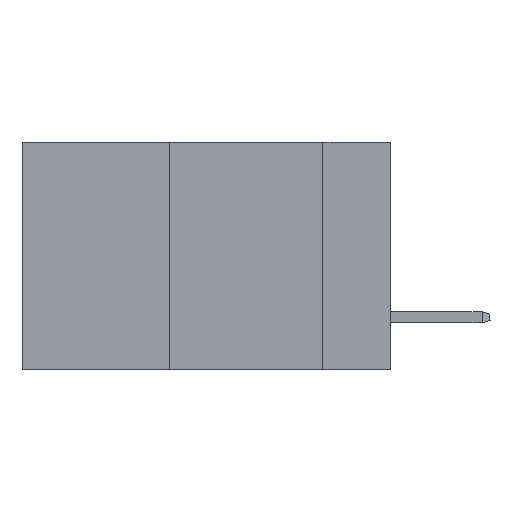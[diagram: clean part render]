
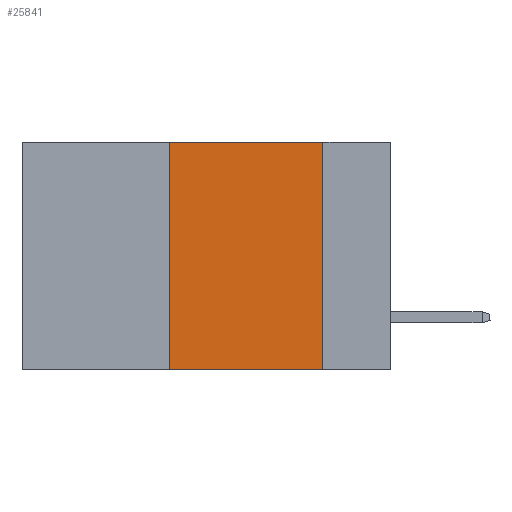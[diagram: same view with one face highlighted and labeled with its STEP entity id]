
A CAD part, left-side view. The second image highlights one B-rep face of the part: STEP entity #25841.
In plain terms, the highlighted planar face has unit normal (-1, 0, 0).
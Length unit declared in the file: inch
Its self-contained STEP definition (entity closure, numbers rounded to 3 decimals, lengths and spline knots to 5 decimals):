
#938 = VECTOR ( 'NONE', #4371, 39.37008 ) ;
#3241 = CARTESIAN_POINT ( 'NONE',  ( 0., 0.36, 0. ) ) ;
#4371 = DIRECTION ( 'NONE',  ( 0., 0., 1. ) ) ;
#6216 = VERTEX_POINT ( 'NONE', #20646 ) ;
#8365 = DIRECTION ( 'NONE',  ( 0., -1., 0. ) ) ;
#10169 = VECTOR ( 'NONE', #24412, 39.37008 ) ;
#11395 = EDGE_CURVE ( 'NONE', #15567, #6216, #29521, .T. ) ;
#13046 = DIRECTION ( 'NONE',  ( 1., 0., 0. ) ) ;
#13505 = VERTEX_POINT ( 'NONE', #3241 ) ;
#14642 = VECTOR ( 'NONE', #37794, 39.37008 ) ;
#14935 = VERTEX_POINT ( 'NONE', #39691 ) ;
#15514 = CARTESIAN_POINT ( 'NONE',  ( 0., 0.6, 0. ) ) ;
#15567 = VERTEX_POINT ( 'NONE', #29729 ) ;
#18575 = EDGE_CURVE ( 'NONE', #14935, #6216, #44314, .T. ) ;
#19691 = VECTOR ( 'NONE', #8365, 39.37008 ) ;
#20646 = CARTESIAN_POINT ( 'NONE',  ( 0., 0.11, -0.37 ) ) ;
#23724 = FACE_OUTER_BOUND ( 'NONE', #37494, .T. ) ;
#24412 = DIRECTION ( 'NONE',  ( 0., -1., 0. ) ) ;
#25841 = ADVANCED_FACE ( 'NONE', ( #23724 ), #41802, .F. ) ;
#29521 = LINE ( 'NONE', #46261, #10169 ) ;
#29678 = CARTESIAN_POINT ( 'NONE',  ( 0., 0.36, 0. ) ) ;
#29729 = CARTESIAN_POINT ( 'NONE',  ( 0., 0.36, -0.37 ) ) ;
#30243 = CARTESIAN_POINT ( 'NONE',  ( 0., 0.11, 0. ) ) ;
#31321 = ORIENTED_EDGE ( 'NONE', *, *, #11395, .T. ) ;
#33709 = ORIENTED_EDGE ( 'NONE', *, *, #39020, .F. ) ;
#34845 = EDGE_CURVE ( 'NONE', #13505, #14935, #40925, .T. ) ;
#37494 = EDGE_LOOP ( 'NONE', ( #37722, #41736, #33709, #31321 ) ) ;
#37722 = ORIENTED_EDGE ( 'NONE', *, *, #18575, .F. ) ;
#37794 = DIRECTION ( 'NONE',  ( 0., 0., -1. ) ) ;
#39020 = EDGE_CURVE ( 'NONE', #15567, #13505, #40318, .T. ) ;
#39691 = CARTESIAN_POINT ( 'NONE',  ( 0., 0.11, 0. ) ) ;
#40318 = LINE ( 'NONE', #29678, #938 ) ;
#40925 = LINE ( 'NONE', #15514, #19691 ) ;
#41736 = ORIENTED_EDGE ( 'NONE', *, *, #34845, .F. ) ;
#41802 = PLANE ( 'NONE',  #45993 ) ;
#42275 = DIRECTION ( 'NONE',  ( 0., 0., -1. ) ) ;
#44314 = LINE ( 'NONE', #30243, #14642 ) ;
#45869 = CARTESIAN_POINT ( 'NONE',  ( 0., 0.6, 0. ) ) ;
#45993 = AXIS2_PLACEMENT_3D ( 'NONE', #45869, #13046, #42275 ) ;
#46261 = CARTESIAN_POINT ( 'NONE',  ( 0., 0.6, -0.37 ) ) ;
